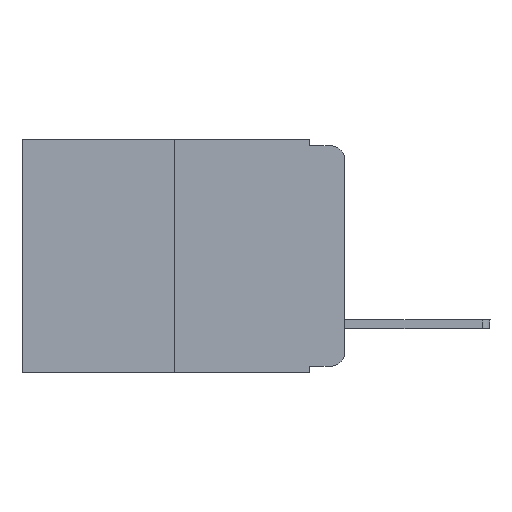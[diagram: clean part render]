
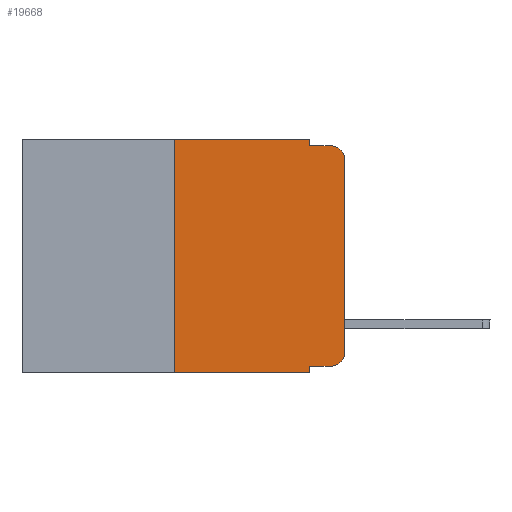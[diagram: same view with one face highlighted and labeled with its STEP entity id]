
A CAD part, left-side view. The second image highlights one B-rep face of the part: STEP entity #19668.
In plain terms, the highlighted planar face has unit normal (-1, 0, 0).
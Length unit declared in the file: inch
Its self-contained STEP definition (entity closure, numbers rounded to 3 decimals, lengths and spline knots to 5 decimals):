
#45 = VERTEX_POINT ( 'NONE', #20350 ) ;
#298 = CIRCLE ( 'NONE', #3394, 0.02 ) ;
#315 = ORIENTED_EDGE ( 'NONE', *, *, #1212, .T. ) ;
#514 = DIRECTION ( 'NONE',  ( 0., 0., 1. ) ) ;
#661 = DIRECTION ( 'NONE',  ( 0., 0., -1. ) ) ;
#704 = EDGE_CURVE ( 'NONE', #10277, #22531, #2131, .T. ) ;
#717 = CARTESIAN_POINT ( 'NONE',  ( 0., 0.051, 0. ) ) ;
#801 = EDGE_CURVE ( 'NONE', #21155, #14902, #15109, .T. ) ;
#1212 = EDGE_CURVE ( 'NONE', #16981, #5997, #22447, .T. ) ;
#1274 = VERTEX_POINT ( 'NONE', #12025 ) ;
#2104 = AXIS2_PLACEMENT_3D ( 'NONE', #13635, #9769, #7831 ) ;
#2131 = LINE ( 'NONE', #13396, #9191 ) ;
#2178 = ORIENTED_EDGE ( 'NONE', *, *, #801, .F. ) ;
#2770 = CIRCLE ( 'NONE', #17107, 0.02 ) ;
#3394 = AXIS2_PLACEMENT_3D ( 'NONE', #4321, #17413, #661 ) ;
#3929 = DIRECTION ( 'NONE',  ( 0., -1., 0. ) ) ;
#4261 = VECTOR ( 'NONE', #22475, 39.37008 ) ;
#4321 = CARTESIAN_POINT ( 'NONE',  ( 0., 0.02, -0.03 ) ) ;
#4323 = PLANE ( 'NONE',  #2104 ) ;
#4481 = VECTOR ( 'NONE', #19814, 39.37008 ) ;
#4669 = ORIENTED_EDGE ( 'NONE', *, *, #15047, .T. ) ;
#5167 = VECTOR ( 'NONE', #17853, 39.37008 ) ;
#5743 = VECTOR ( 'NONE', #11651, 39.37008 ) ;
#5997 = VERTEX_POINT ( 'NONE', #19672 ) ;
#6194 = ORIENTED_EDGE ( 'NONE', *, *, #22584, .T. ) ;
#6211 = LINE ( 'NONE', #7687, #21964 ) ;
#6564 = LINE ( 'NONE', #12399, #5167 ) ;
#7229 = CARTESIAN_POINT ( 'NONE',  ( 0., 0.051, -0.01 ) ) ;
#7262 = DIRECTION ( 'NONE',  ( -1., 0., 0. ) ) ;
#7342 = EDGE_CURVE ( 'NONE', #16981, #1274, #18013, .T. ) ;
#7634 = ORIENTED_EDGE ( 'NONE', *, *, #704, .F. ) ;
#7687 = CARTESIAN_POINT ( 'NONE',  ( 0., 0.25, 0. ) ) ;
#7831 = DIRECTION ( 'NONE',  ( 0., 0., -1. ) ) ;
#7937 = DIRECTION ( 'NONE',  ( 0., -1., 0. ) ) ;
#8003 = LINE ( 'NONE', #717, #5743 ) ;
#8061 = VECTOR ( 'NONE', #18260, 39.37008 ) ;
#9191 = VECTOR ( 'NONE', #7937, 39.37008 ) ;
#9769 = DIRECTION ( 'NONE',  ( 1., 0., 0. ) ) ;
#10079 = ORIENTED_EDGE ( 'NONE', *, *, #7342, .F. ) ;
#10277 = VERTEX_POINT ( 'NONE', #7229 ) ;
#10303 = EDGE_CURVE ( 'NONE', #45, #1274, #21887, .T. ) ;
#10906 = DIRECTION ( 'NONE',  ( 0., 0., -1. ) ) ;
#11322 = VECTOR ( 'NONE', #3929, 39.37008 ) ;
#11376 = EDGE_CURVE ( 'NONE', #14902, #10277, #8003, .T. ) ;
#11651 = DIRECTION ( 'NONE',  ( 0., 0., -1. ) ) ;
#11718 = FACE_OUTER_BOUND ( 'NONE', #21695, .T. ) ;
#12025 = CARTESIAN_POINT ( 'NONE',  ( 0., 0.051, -0.343 ) ) ;
#12342 = VERTEX_POINT ( 'NONE', #18329 ) ;
#12399 = CARTESIAN_POINT ( 'NONE',  ( 0., 0., 0. ) ) ;
#12807 = CARTESIAN_POINT ( 'NONE',  ( 0., 0.051, 0. ) ) ;
#13280 = CARTESIAN_POINT ( 'NONE',  ( 0., 0.473, 0. ) ) ;
#13396 = CARTESIAN_POINT ( 'NONE',  ( 0., 0.051, -0.01 ) ) ;
#13519 = CARTESIAN_POINT ( 'NONE',  ( 0., 0.02, -0.01 ) ) ;
#13635 = CARTESIAN_POINT ( 'NONE',  ( 0., 0.473, 0. ) ) ;
#14894 = ORIENTED_EDGE ( 'NONE', *, *, #11376, .F. ) ;
#14902 = VERTEX_POINT ( 'NONE', #19053 ) ;
#15047 = EDGE_CURVE ( 'NONE', #5997, #20092, #2770, .T. ) ;
#15109 = LINE ( 'NONE', #13280, #4261 ) ;
#16036 = ORIENTED_EDGE ( 'NONE', *, *, #17386, .T. ) ;
#16981 = VERTEX_POINT ( 'NONE', #20049 ) ;
#17107 = AXIS2_PLACEMENT_3D ( 'NONE', #19859, #7262, #10906 ) ;
#17217 = CARTESIAN_POINT ( 'NONE',  ( 0., 0.25, 0. ) ) ;
#17386 = EDGE_CURVE ( 'NONE', #20092, #12342, #6564, .T. ) ;
#17413 = DIRECTION ( 'NONE',  ( -1., 0., 0. ) ) ;
#17853 = DIRECTION ( 'NONE',  ( 0., 0., 1. ) ) ;
#18013 = LINE ( 'NONE', #12807, #4481 ) ;
#18053 = ORIENTED_EDGE ( 'NONE', *, *, #23043, .F. ) ;
#18260 = DIRECTION ( 'NONE',  ( 0., -1., 0. ) ) ;
#18329 = CARTESIAN_POINT ( 'NONE',  ( 0., 0., -0.03 ) ) ;
#18840 = CARTESIAN_POINT ( 'NONE',  ( 0., 0., -0.313 ) ) ;
#18948 = CARTESIAN_POINT ( 'NONE',  ( 0., 0.051, -0.333 ) ) ;
#19053 = CARTESIAN_POINT ( 'NONE',  ( 0., 0.051, 0. ) ) ;
#19668 = ADVANCED_FACE ( 'NONE', ( #11718 ), #4323, .F. ) ;
#19672 = CARTESIAN_POINT ( 'NONE',  ( 0., 0.02, -0.333 ) ) ;
#19814 = DIRECTION ( 'NONE',  ( 0., 0., -1. ) ) ;
#19859 = CARTESIAN_POINT ( 'NONE',  ( 0., 0.02, -0.313 ) ) ;
#20049 = CARTESIAN_POINT ( 'NONE',  ( 0., 0.051, -0.333 ) ) ;
#20092 = VERTEX_POINT ( 'NONE', #18840 ) ;
#20350 = CARTESIAN_POINT ( 'NONE',  ( 0., 0.25, -0.343 ) ) ;
#21155 = VERTEX_POINT ( 'NONE', #17217 ) ;
#21695 = EDGE_LOOP ( 'NONE', ( #16036, #6194, #7634, #14894, #2178, #18053, #22287, #10079, #315, #4669 ) ) ;
#21887 = LINE ( 'NONE', #23702, #8061 ) ;
#21964 = VECTOR ( 'NONE', #514, 39.37008 ) ;
#22287 = ORIENTED_EDGE ( 'NONE', *, *, #10303, .T. ) ;
#22447 = LINE ( 'NONE', #18948, #11322 ) ;
#22475 = DIRECTION ( 'NONE',  ( 0., -1., 0. ) ) ;
#22531 = VERTEX_POINT ( 'NONE', #13519 ) ;
#22584 = EDGE_CURVE ( 'NONE', #12342, #22531, #298, .T. ) ;
#23043 = EDGE_CURVE ( 'NONE', #45, #21155, #6211, .T. ) ;
#23702 = CARTESIAN_POINT ( 'NONE',  ( 0., 0.473, -0.343 ) ) ;
